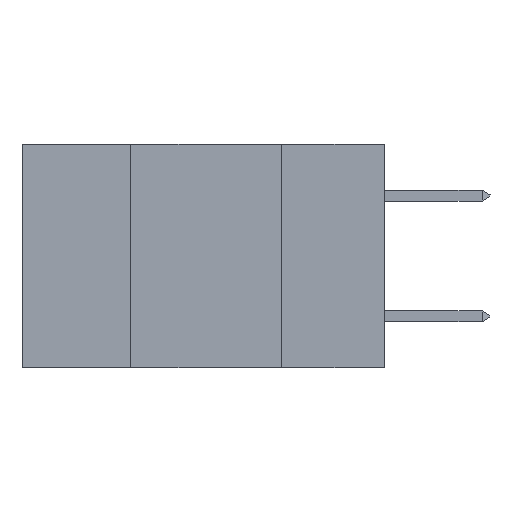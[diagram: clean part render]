
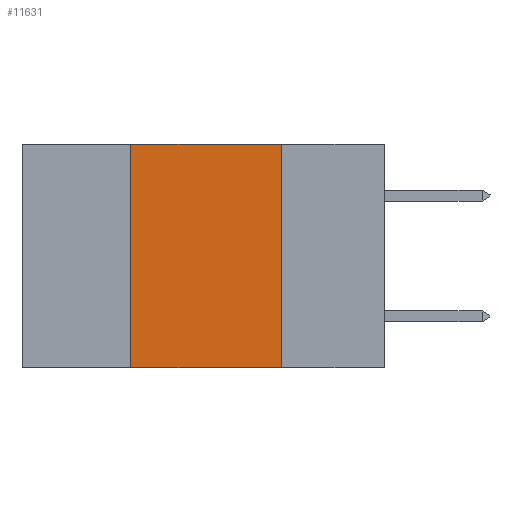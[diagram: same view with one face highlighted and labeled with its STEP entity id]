
A CAD part, left-side view. The second image highlights one B-rep face of the part: STEP entity #11631.
In plain terms, the highlighted planar face has unit normal (-1, 0, 0).
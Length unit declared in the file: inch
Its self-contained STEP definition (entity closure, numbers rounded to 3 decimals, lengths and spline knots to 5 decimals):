
#173 = CARTESIAN_POINT ( 'NONE',  ( 0., 0.17, 0. ) ) ;
#670 = ORIENTED_EDGE ( 'NONE', *, *, #6932, .F. ) ;
#1481 = FACE_OUTER_BOUND ( 'NONE', #22458, .T. ) ;
#4013 = CARTESIAN_POINT ( 'NONE',  ( 0., 0.6, -0.37 ) ) ;
#5678 = CARTESIAN_POINT ( 'NONE',  ( 0., 0.17, 0. ) ) ;
#5900 = DIRECTION ( 'NONE',  ( 0., 0., -1. ) ) ;
#6185 = VERTEX_POINT ( 'NONE', #173 ) ;
#6932 = EDGE_CURVE ( 'NONE', #13937, #19101, #22395, .T. ) ;
#7421 = DIRECTION ( 'NONE',  ( 0., 0., 1. ) ) ;
#7568 = VECTOR ( 'NONE', #9024, 39.37008 ) ;
#7743 = LINE ( 'NONE', #20759, #22709 ) ;
#7848 = DIRECTION ( 'NONE',  ( 1., 0., 0. ) ) ;
#8651 = EDGE_CURVE ( 'NONE', #19101, #6185, #7743, .T. ) ;
#9024 = DIRECTION ( 'NONE',  ( 0., -1., 0. ) ) ;
#10265 = CARTESIAN_POINT ( 'NONE',  ( 0., 0.42, 0. ) ) ;
#11631 = ADVANCED_FACE ( 'NONE', ( #1481 ), #12076, .F. ) ;
#12076 = PLANE ( 'NONE',  #12887 ) ;
#12887 = AXIS2_PLACEMENT_3D ( 'NONE', #14829, #7848, #12926 ) ;
#12926 = DIRECTION ( 'NONE',  ( 0., 0., -1. ) ) ;
#13200 = DIRECTION ( 'NONE',  ( 0., -1., 0. ) ) ;
#13937 = VERTEX_POINT ( 'NONE', #31469 ) ;
#14780 = EDGE_CURVE ( 'NONE', #13937, #17164, #25996, .T. ) ;
#14829 = CARTESIAN_POINT ( 'NONE',  ( 0., 0.6, 0. ) ) ;
#16060 = VECTOR ( 'NONE', #7421, 39.37008 ) ;
#17164 = VERTEX_POINT ( 'NONE', #21133 ) ;
#17784 = EDGE_CURVE ( 'NONE', #6185, #17164, #27267, .T. ) ;
#19101 = VERTEX_POINT ( 'NONE', #26146 ) ;
#19173 = ORIENTED_EDGE ( 'NONE', *, *, #14780, .T. ) ;
#20759 = CARTESIAN_POINT ( 'NONE',  ( 0., 0.6, 0. ) ) ;
#21133 = CARTESIAN_POINT ( 'NONE',  ( 0., 0.17, -0.37 ) ) ;
#22395 = LINE ( 'NONE', #10265, #16060 ) ;
#22458 = EDGE_LOOP ( 'NONE', ( #28840, #23755, #670, #19173 ) ) ;
#22709 = VECTOR ( 'NONE', #13200, 39.37008 ) ;
#23755 = ORIENTED_EDGE ( 'NONE', *, *, #8651, .F. ) ;
#25996 = LINE ( 'NONE', #4013, #7568 ) ;
#26146 = CARTESIAN_POINT ( 'NONE',  ( 0., 0.42, 0. ) ) ;
#26467 = VECTOR ( 'NONE', #5900, 39.37008 ) ;
#27267 = LINE ( 'NONE', #5678, #26467 ) ;
#28840 = ORIENTED_EDGE ( 'NONE', *, *, #17784, .F. ) ;
#31469 = CARTESIAN_POINT ( 'NONE',  ( 0., 0.42, -0.37 ) ) ;
